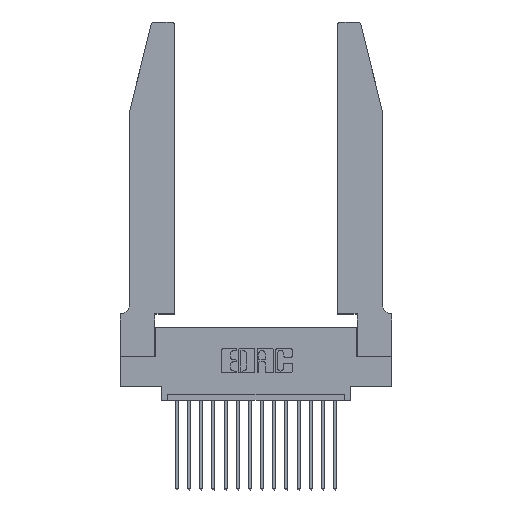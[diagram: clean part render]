
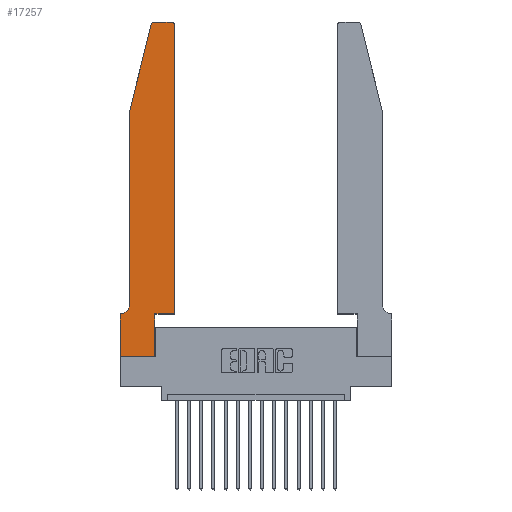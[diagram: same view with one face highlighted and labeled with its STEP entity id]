
A CAD part, top view. The second image highlights one B-rep face of the part: STEP entity #17257.
In plain terms, the highlighted planar face has unit normal (0, 0, 1).
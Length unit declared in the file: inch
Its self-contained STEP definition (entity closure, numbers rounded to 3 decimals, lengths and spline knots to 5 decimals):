
#136 = CARTESIAN_POINT ( 'NONE',  ( 0.0055, 0.35, 0.37 ) ) ;
#289 = CARTESIAN_POINT ( 'NONE',  ( 0.0755, 0.35, 0.37 ) ) ;
#310 = DIRECTION ( 'NONE',  ( 0., 0., 1. ) ) ;
#318 = AXIS2_PLACEMENT_3D ( 'NONE', #12154, #13375, #17923 ) ;
#492 = VECTOR ( 'NONE', #10411, 39.37008 ) ;
#502 = DIRECTION ( 'NONE',  ( 0., 0., -1. ) ) ;
#786 = ORIENTED_EDGE ( 'NONE', *, *, #12160, .T. ) ;
#799 = VECTOR ( 'NONE', #11759, 39.37008 ) ;
#992 = VERTEX_POINT ( 'NONE', #14277 ) ;
#1372 = VECTOR ( 'NONE', #3792, 39.37008 ) ;
#1549 = CARTESIAN_POINT ( 'NONE',  ( 0.2865, 0.35, 0.37 ) ) ;
#1556 = EDGE_CURVE ( 'NONE', #6939, #992, #5584, .T. ) ;
#1914 = DIRECTION ( 'NONE',  ( 1., 0., 0. ) ) ;
#2091 = DIRECTION ( 'NONE',  ( -1., 0., 0. ) ) ;
#2626 = VERTEX_POINT ( 'NONE', #16160 ) ;
#2711 = CARTESIAN_POINT ( 'NONE',  ( 0.4505, 2.72, 0.37 ) ) ;
#2712 = ORIENTED_EDGE ( 'NONE', *, *, #18606, .T. ) ;
#3049 = DIRECTION ( 'NONE',  ( 0., 1., 0. ) ) ;
#3121 = VECTOR ( 'NONE', #1914, 39.37008 ) ;
#3183 = VERTEX_POINT ( 'NONE', #18919 ) ;
#3557 = ORIENTED_EDGE ( 'NONE', *, *, #8022, .T. ) ;
#3574 = VERTEX_POINT ( 'NONE', #10773 ) ;
#3792 = DIRECTION ( 'NONE',  ( -1., 0., 0. ) ) ;
#4751 = CARTESIAN_POINT ( 'NONE',  ( 0.2865, 0., 0.37 ) ) ;
#4928 = VECTOR ( 'NONE', #7764, 39.37008 ) ;
#5165 = DIRECTION ( 'NONE',  ( -1., 0., 0. ) ) ;
#5194 = CARTESIAN_POINT ( 'NONE',  ( 0., 0., 0.37 ) ) ;
#5508 = VECTOR ( 'NONE', #3049, 39.37008 ) ;
#5572 = ORIENTED_EDGE ( 'NONE', *, *, #14967, .T. ) ;
#5584 = LINE ( 'NONE', #11494, #13693 ) ;
#6107 = ORIENTED_EDGE ( 'NONE', *, *, #13614, .T. ) ;
#6354 = EDGE_LOOP ( 'NONE', ( #5572, #14921, #18610, #11843, #8430, #6107, #8153, #786, #16639, #2712, #3557, #12923 ) ) ;
#6563 = VECTOR ( 'NONE', #17176, 39.37008 ) ;
#6939 = VERTEX_POINT ( 'NONE', #11836 ) ;
#7406 = CIRCLE ( 'NONE', #15531, 0.03 ) ;
#7764 = DIRECTION ( 'NONE',  ( 0., 1., 0. ) ) ;
#8022 = EDGE_CURVE ( 'NONE', #11805, #17017, #11377, .T. ) ;
#8041 = CARTESIAN_POINT ( 'NONE',  ( 0.4205, 2.72, 0.37 ) ) ;
#8153 = ORIENTED_EDGE ( 'NONE', *, *, #8607, .T. ) ;
#8188 = FACE_OUTER_BOUND ( 'NONE', #6354, .T. ) ;
#8306 = VERTEX_POINT ( 'NONE', #13689 ) ;
#8430 = ORIENTED_EDGE ( 'NONE', *, *, #9920, .T. ) ;
#8607 = EDGE_CURVE ( 'NONE', #8306, #2626, #10471, .T. ) ;
#9081 = LINE ( 'NONE', #5194, #6563 ) ;
#9199 = PLANE ( 'NONE',  #13085 ) ;
#9269 = CARTESIAN_POINT ( 'NONE',  ( 0., 0.35, 0.37 ) ) ;
#9920 = EDGE_CURVE ( 'NONE', #992, #15404, #11569, .T. ) ;
#10328 = CARTESIAN_POINT ( 'NONE',  ( 0.0755, 2., 0.37 ) ) ;
#10411 = DIRECTION ( 'NONE',  ( 0., -1., 0. ) ) ;
#10471 = LINE ( 'NONE', #16179, #492 ) ;
#10773 = CARTESIAN_POINT ( 'NONE',  ( 0.25487, 2.72718, 0.37 ) ) ;
#10836 = LINE ( 'NONE', #1549, #5508 ) ;
#11041 = CARTESIAN_POINT ( 'NONE',  ( 0.0055, 0.42, 0.37 ) ) ;
#11215 = EDGE_CURVE ( 'NONE', #19077, #3183, #10836, .T. ) ;
#11371 = LINE ( 'NONE', #289, #19045 ) ;
#11377 = LINE ( 'NONE', #12147, #4928 ) ;
#11494 = CARTESIAN_POINT ( 'NONE',  ( 0.0755, 2., 0.37 ) ) ;
#11569 = CIRCLE ( 'NONE', #17744, 0.07 ) ;
#11759 = DIRECTION ( 'NONE',  ( -0.239, -0.971, 0. ) ) ;
#11805 = VERTEX_POINT ( 'NONE', #12171 ) ;
#11836 = CARTESIAN_POINT ( 'NONE',  ( 0.0755, 2., 0.37 ) ) ;
#11843 = ORIENTED_EDGE ( 'NONE', *, *, #1556, .T. ) ;
#12147 = CARTESIAN_POINT ( 'NONE',  ( 0.4505, 0.35, 0.37 ) ) ;
#12154 = CARTESIAN_POINT ( 'NONE',  ( 0.284, 2.72, 0.37 ) ) ;
#12160 = EDGE_CURVE ( 'NONE', #2626, #19077, #9081, .T. ) ;
#12171 = CARTESIAN_POINT ( 'NONE',  ( 0.4505, 0.35, 0.37 ) ) ;
#12376 = DIRECTION ( 'NONE',  ( 1., 0., 0. ) ) ;
#12678 = DIRECTION ( 'NONE',  ( 1., 0., 0. ) ) ;
#12923 = ORIENTED_EDGE ( 'NONE', *, *, #14626, .T. ) ;
#13085 = AXIS2_PLACEMENT_3D ( 'NONE', #9269, #310, #12376 ) ;
#13202 = LINE ( 'NONE', #18685, #1372 ) ;
#13228 = VERTEX_POINT ( 'NONE', #14426 ) ;
#13375 = DIRECTION ( 'NONE',  ( 0., 0., 1. ) ) ;
#13614 = EDGE_CURVE ( 'NONE', #15404, #8306, #11371, .T. ) ;
#13689 = CARTESIAN_POINT ( 'NONE',  ( 0., 0.35, 0.37 ) ) ;
#13693 = VECTOR ( 'NONE', #16259, 39.37008 ) ;
#14277 = CARTESIAN_POINT ( 'NONE',  ( 0.0755, 0.42, 0.37 ) ) ;
#14426 = CARTESIAN_POINT ( 'NONE',  ( 0.4205, 2.75, 0.37 ) ) ;
#14576 = CARTESIAN_POINT ( 'NONE',  ( 0.284, 2.75, 0.37 ) ) ;
#14626 = EDGE_CURVE ( 'NONE', #17017, #13228, #7406, .T. ) ;
#14921 = ORIENTED_EDGE ( 'NONE', *, *, #17835, .T. ) ;
#14967 = EDGE_CURVE ( 'NONE', #13228, #18893, #13202, .T. ) ;
#15404 = VERTEX_POINT ( 'NONE', #136 ) ;
#15511 = DIRECTION ( 'NONE',  ( 0., 0., 1. ) ) ;
#15531 = AXIS2_PLACEMENT_3D ( 'NONE', #8041, #15511, #12678 ) ;
#16160 = CARTESIAN_POINT ( 'NONE',  ( 0., 0., 0.37 ) ) ;
#16179 = CARTESIAN_POINT ( 'NONE',  ( 0., 0., 0.37 ) ) ;
#16259 = DIRECTION ( 'NONE',  ( 0., -1., 0. ) ) ;
#16564 = LINE ( 'NONE', #10328, #799 ) ;
#16639 = ORIENTED_EDGE ( 'NONE', *, *, #11215, .T. ) ;
#16742 = CARTESIAN_POINT ( 'NONE',  ( 0.4505, 0.35, 0.37 ) ) ;
#17017 = VERTEX_POINT ( 'NONE', #2711 ) ;
#17176 = DIRECTION ( 'NONE',  ( 1., 0., 0. ) ) ;
#17257 = ADVANCED_FACE ( 'NONE', ( #8188 ), #9199, .T. ) ;
#17744 = AXIS2_PLACEMENT_3D ( 'NONE', #11041, #502, #5165 ) ;
#17835 = EDGE_CURVE ( 'NONE', #18893, #3574, #18664, .T. ) ;
#17923 = DIRECTION ( 'NONE',  ( 1., 0., 0. ) ) ;
#18357 = EDGE_CURVE ( 'NONE', #3574, #6939, #16564, .T. ) ;
#18606 = EDGE_CURVE ( 'NONE', #3183, #11805, #18874, .T. ) ;
#18610 = ORIENTED_EDGE ( 'NONE', *, *, #18357, .T. ) ;
#18664 = CIRCLE ( 'NONE', #318, 0.03 ) ;
#18685 = CARTESIAN_POINT ( 'NONE',  ( 0.2605, 2.75, 0.37 ) ) ;
#18874 = LINE ( 'NONE', #16742, #3121 ) ;
#18893 = VERTEX_POINT ( 'NONE', #14576 ) ;
#18919 = CARTESIAN_POINT ( 'NONE',  ( 0.2865, 0.35, 0.37 ) ) ;
#19045 = VECTOR ( 'NONE', #2091, 39.37008 ) ;
#19077 = VERTEX_POINT ( 'NONE', #4751 ) ;
